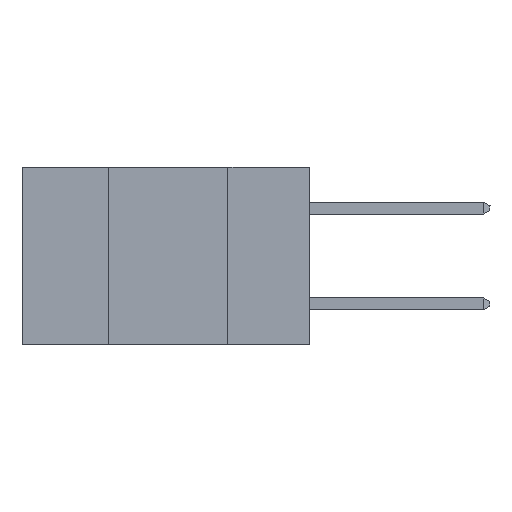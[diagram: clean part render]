
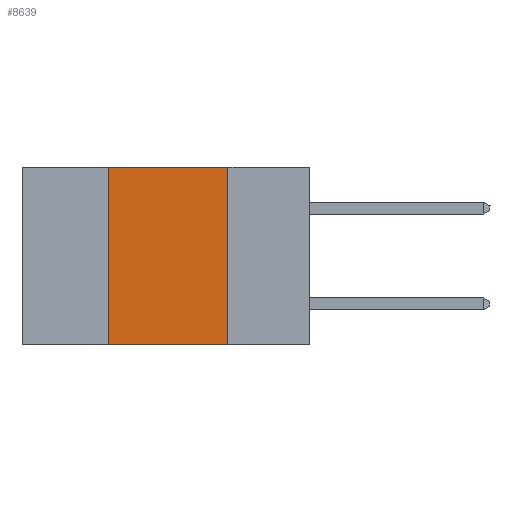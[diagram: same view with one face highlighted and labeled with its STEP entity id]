
A CAD part, left-side view. The second image highlights one B-rep face of the part: STEP entity #8639.
In plain terms, the highlighted planar face has unit normal (-1, 0, 0).
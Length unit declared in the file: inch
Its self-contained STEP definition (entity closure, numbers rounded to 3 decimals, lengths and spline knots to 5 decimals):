
#575 = DIRECTION ( 'NONE',  ( 0., -1., 0. ) ) ;
#763 = EDGE_CURVE ( 'NONE', #18799, #9814, #1252, .T. ) ;
#1206 = CARTESIAN_POINT ( 'NONE',  ( 0., 0.17, 0. ) ) ;
#1252 = LINE ( 'NONE', #16870, #2727 ) ;
#1535 = DIRECTION ( 'NONE',  ( 0., -1., 0. ) ) ;
#1718 = EDGE_LOOP ( 'NONE', ( #5263, #10123, #3409, #10355 ) ) ;
#1719 = EDGE_CURVE ( 'NONE', #16920, #18491, #11975, .T. ) ;
#2171 = PLANE ( 'NONE',  #18619 ) ;
#2727 = VECTOR ( 'NONE', #1535, 39.37008 ) ;
#2956 = LINE ( 'NONE', #12352, #6654 ) ;
#3409 = ORIENTED_EDGE ( 'NONE', *, *, #18368, .F. ) ;
#3883 = DIRECTION ( 'NONE',  ( 1., 0., 0. ) ) ;
#5263 = ORIENTED_EDGE ( 'NONE', *, *, #9822, .F. ) ;
#6654 = VECTOR ( 'NONE', #16898, 39.37008 ) ;
#6733 = LINE ( 'NONE', #12267, #10615 ) ;
#8639 = ADVANCED_FACE ( 'NONE', ( #10680 ), #2171, .F. ) ;
#9814 = VERTEX_POINT ( 'NONE', #1206 ) ;
#9822 = EDGE_CURVE ( 'NONE', #9814, #18491, #6733, .T. ) ;
#10005 = DIRECTION ( 'NONE',  ( 0., 0., -1. ) ) ;
#10123 = ORIENTED_EDGE ( 'NONE', *, *, #763, .F. ) ;
#10355 = ORIENTED_EDGE ( 'NONE', *, *, #1719, .T. ) ;
#10615 = VECTOR ( 'NONE', #20107, 39.37008 ) ;
#10680 = FACE_OUTER_BOUND ( 'NONE', #1718, .T. ) ;
#11975 = LINE ( 'NONE', #16348, #19707 ) ;
#12267 = CARTESIAN_POINT ( 'NONE',  ( 0., 0.17, 0. ) ) ;
#12352 = CARTESIAN_POINT ( 'NONE',  ( 0., 0.42, 0. ) ) ;
#12729 = CARTESIAN_POINT ( 'NONE',  ( 0., 0.17, -0.37 ) ) ;
#13089 = CARTESIAN_POINT ( 'NONE',  ( 0., 0.6, 0. ) ) ;
#16348 = CARTESIAN_POINT ( 'NONE',  ( 0., 0.6, -0.37 ) ) ;
#16870 = CARTESIAN_POINT ( 'NONE',  ( 0., 0.6, 0. ) ) ;
#16898 = DIRECTION ( 'NONE',  ( 0., 0., 1. ) ) ;
#16920 = VERTEX_POINT ( 'NONE', #19417 ) ;
#18368 = EDGE_CURVE ( 'NONE', #16920, #18799, #2956, .T. ) ;
#18491 = VERTEX_POINT ( 'NONE', #12729 ) ;
#18619 = AXIS2_PLACEMENT_3D ( 'NONE', #13089, #3883, #10005 ) ;
#18799 = VERTEX_POINT ( 'NONE', #19521 ) ;
#19417 = CARTESIAN_POINT ( 'NONE',  ( 0., 0.42, -0.37 ) ) ;
#19521 = CARTESIAN_POINT ( 'NONE',  ( 0., 0.42, 0. ) ) ;
#19707 = VECTOR ( 'NONE', #575, 39.37008 ) ;
#20107 = DIRECTION ( 'NONE',  ( 0., 0., -1. ) ) ;
